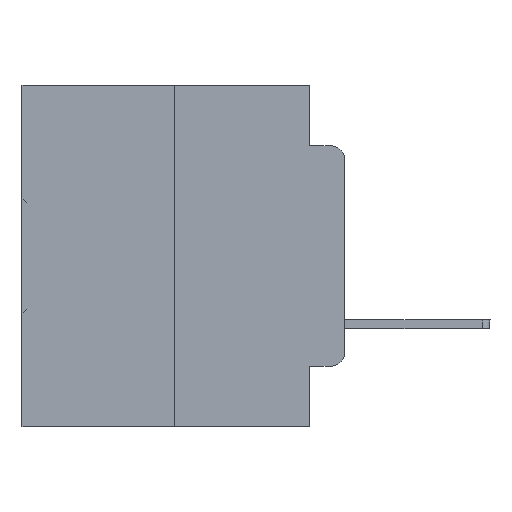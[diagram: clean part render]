
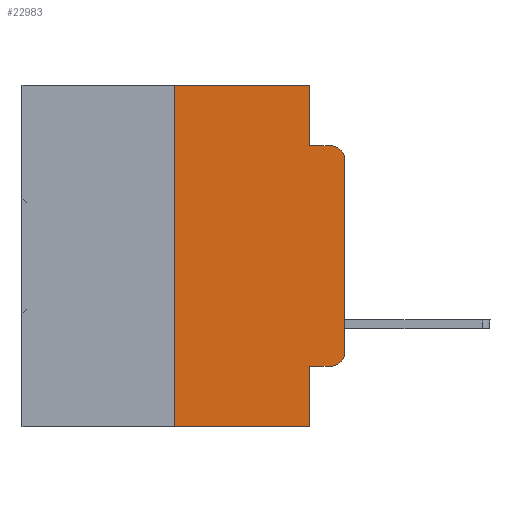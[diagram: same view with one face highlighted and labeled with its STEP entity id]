
A CAD part, left-side view. The second image highlights one B-rep face of the part: STEP entity #22983.
In plain terms, the highlighted planar face has unit normal (-1, 0, 0).
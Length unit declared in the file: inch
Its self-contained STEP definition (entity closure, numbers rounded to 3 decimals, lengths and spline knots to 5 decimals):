
#268 = EDGE_CURVE ( 'NONE', #5514, #24024, #1679, .T. ) ;
#509 = DIRECTION ( 'NONE',  ( 0., 0., -1. ) ) ;
#887 = LINE ( 'NONE', #2048, #8177 ) ;
#1679 = LINE ( 'NONE', #31376, #31170 ) ;
#2048 = CARTESIAN_POINT ( 'NONE',  ( 0., 0., 0. ) ) ;
#2562 = DIRECTION ( 'NONE',  ( 0., 0., -1. ) ) ;
#2893 = CARTESIAN_POINT ( 'NONE',  ( 0., 0.051, -0.4115 ) ) ;
#2985 = ORIENTED_EDGE ( 'NONE', *, *, #20421, .T. ) ;
#3041 = LINE ( 'NONE', #6475, #20890 ) ;
#3155 = ORIENTED_EDGE ( 'NONE', *, *, #7954, .T. ) ;
#4027 = VECTOR ( 'NONE', #32027, 39.37008 ) ;
#4044 = DIRECTION ( 'NONE',  ( -1., 0., 0. ) ) ;
#4192 = CARTESIAN_POINT ( 'NONE',  ( 0., 0.02, -0.4115 ) ) ;
#4312 = EDGE_LOOP ( 'NONE', ( #26978, #26481, #26988, #32103, #28508, #13017, #18344, #31179, #2985, #3155 ) ) ;
#4773 = CIRCLE ( 'NONE', #26028, 0.02 ) ;
#4840 = LINE ( 'NONE', #19065, #4027 ) ;
#5141 = EDGE_CURVE ( 'NONE', #24024, #20112, #23118, .T. ) ;
#5305 = VERTEX_POINT ( 'NONE', #19238 ) ;
#5514 = VERTEX_POINT ( 'NONE', #31022 ) ;
#5674 = DIRECTION ( 'NONE',  ( 0., -1., 0. ) ) ;
#5783 = DIRECTION ( 'NONE',  ( 0., 0., 1. ) ) ;
#5850 = CARTESIAN_POINT ( 'NONE',  ( 0., 0.02, -0.3915 ) ) ;
#6118 = EDGE_CURVE ( 'NONE', #5305, #20112, #31885, .T. ) ;
#6475 = CARTESIAN_POINT ( 'NONE',  ( 0., 0.473, -0.5 ) ) ;
#7050 = EDGE_CURVE ( 'NONE', #13968, #5514, #4840, .T. ) ;
#7954 = EDGE_CURVE ( 'NONE', #12709, #11033, #4773, .T. ) ;
#8047 = CARTESIAN_POINT ( 'NONE',  ( 0., 0.25, 0. ) ) ;
#8177 = VECTOR ( 'NONE', #18747, 39.37008 ) ;
#8423 = EDGE_CURVE ( 'NONE', #22383, #13968, #27733, .T. ) ;
#8475 = AXIS2_PLACEMENT_3D ( 'NONE', #32159, #4044, #16689 ) ;
#8788 = DIRECTION ( 'NONE',  ( -1., 0., 0. ) ) ;
#9174 = CARTESIAN_POINT ( 'NONE',  ( 0., 0.25, -0.5 ) ) ;
#9500 = VECTOR ( 'NONE', #2562, 39.37008 ) ;
#10061 = CARTESIAN_POINT ( 'NONE',  ( 0., 0.051, -0.4115 ) ) ;
#11033 = VERTEX_POINT ( 'NONE', #24238 ) ;
#11619 = DIRECTION ( 'NONE',  ( 0., -1., 0. ) ) ;
#11676 = CARTESIAN_POINT ( 'NONE',  ( 0., 0.02, -0.0885 ) ) ;
#12709 = VERTEX_POINT ( 'NONE', #4192 ) ;
#12813 = CARTESIAN_POINT ( 'NONE',  ( 0., 0.051, 0. ) ) ;
#13017 = ORIENTED_EDGE ( 'NONE', *, *, #8423, .F. ) ;
#13079 = VECTOR ( 'NONE', #32143, 39.37008 ) ;
#13348 = FACE_OUTER_BOUND ( 'NONE', #4312, .T. ) ;
#13738 = VECTOR ( 'NONE', #5674, 39.37008 ) ;
#13968 = VERTEX_POINT ( 'NONE', #22393 ) ;
#14999 = VERTEX_POINT ( 'NONE', #10061 ) ;
#16689 = DIRECTION ( 'NONE',  ( 0., 0., -1. ) ) ;
#16829 = DIRECTION ( 'NONE',  ( 0., 0., -1. ) ) ;
#16949 = PLANE ( 'NONE',  #18545 ) ;
#18344 = ORIENTED_EDGE ( 'NONE', *, *, #25982, .T. ) ;
#18370 = LINE ( 'NONE', #12813, #9500 ) ;
#18545 = AXIS2_PLACEMENT_3D ( 'NONE', #26944, #29784, #16829 ) ;
#18747 = DIRECTION ( 'NONE',  ( 0., 0., 1. ) ) ;
#19065 = CARTESIAN_POINT ( 'NONE',  ( 0., 0.473, 0. ) ) ;
#19238 = CARTESIAN_POINT ( 'NONE',  ( 0., 0., -0.1085 ) ) ;
#20112 = VERTEX_POINT ( 'NONE', #11676 ) ;
#20421 = EDGE_CURVE ( 'NONE', #14999, #12709, #22847, .T. ) ;
#20622 = CARTESIAN_POINT ( 'NONE',  ( 0., 0.051, -0.0885 ) ) ;
#20890 = VECTOR ( 'NONE', #11619, 39.37008 ) ;
#21280 = VECTOR ( 'NONE', #5783, 39.37008 ) ;
#22383 = VERTEX_POINT ( 'NONE', #9174 ) ;
#22393 = CARTESIAN_POINT ( 'NONE',  ( 0., 0.25, 0. ) ) ;
#22847 = LINE ( 'NONE', #2893, #13079 ) ;
#22983 = ADVANCED_FACE ( 'NONE', ( #13348 ), #16949, .F. ) ;
#23118 = LINE ( 'NONE', #26540, #13738 ) ;
#24024 = VERTEX_POINT ( 'NONE', #20622 ) ;
#24238 = CARTESIAN_POINT ( 'NONE',  ( 0., 0., -0.3915 ) ) ;
#25982 = EDGE_CURVE ( 'NONE', #22383, #27974, #3041, .T. ) ;
#26028 = AXIS2_PLACEMENT_3D ( 'NONE', #5850, #8788, #509 ) ;
#26481 = ORIENTED_EDGE ( 'NONE', *, *, #6118, .T. ) ;
#26540 = CARTESIAN_POINT ( 'NONE',  ( 0., 0.051, -0.0885 ) ) ;
#26690 = CARTESIAN_POINT ( 'NONE',  ( 0., 0.051, -0.5 ) ) ;
#26944 = CARTESIAN_POINT ( 'NONE',  ( 0., 0.473, 0. ) ) ;
#26978 = ORIENTED_EDGE ( 'NONE', *, *, #30876, .T. ) ;
#26988 = ORIENTED_EDGE ( 'NONE', *, *, #5141, .F. ) ;
#27733 = LINE ( 'NONE', #8047, #21280 ) ;
#27974 = VERTEX_POINT ( 'NONE', #26690 ) ;
#28508 = ORIENTED_EDGE ( 'NONE', *, *, #7050, .F. ) ;
#28872 = DIRECTION ( 'NONE',  ( 0., 0., -1. ) ) ;
#29604 = EDGE_CURVE ( 'NONE', #14999, #27974, #18370, .T. ) ;
#29784 = DIRECTION ( 'NONE',  ( 1., 0., 0. ) ) ;
#30876 = EDGE_CURVE ( 'NONE', #11033, #5305, #887, .T. ) ;
#31022 = CARTESIAN_POINT ( 'NONE',  ( 0., 0.051, 0. ) ) ;
#31170 = VECTOR ( 'NONE', #28872, 39.37008 ) ;
#31179 = ORIENTED_EDGE ( 'NONE', *, *, #29604, .F. ) ;
#31376 = CARTESIAN_POINT ( 'NONE',  ( 0., 0.051, 0. ) ) ;
#31885 = CIRCLE ( 'NONE', #8475, 0.02 ) ;
#32027 = DIRECTION ( 'NONE',  ( 0., -1., 0. ) ) ;
#32103 = ORIENTED_EDGE ( 'NONE', *, *, #268, .F. ) ;
#32143 = DIRECTION ( 'NONE',  ( 0., -1., 0. ) ) ;
#32159 = CARTESIAN_POINT ( 'NONE',  ( 0., 0.02, -0.1085 ) ) ;
